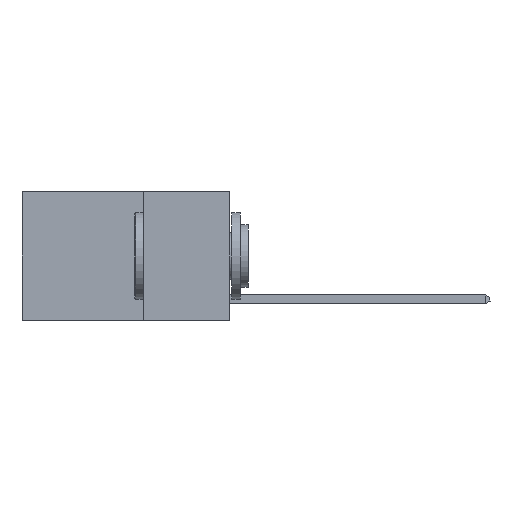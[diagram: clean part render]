
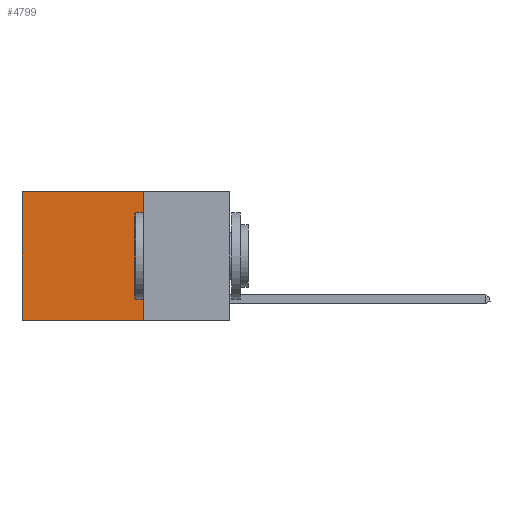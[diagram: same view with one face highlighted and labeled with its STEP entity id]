
A CAD part, left-side view. The second image highlights one B-rep face of the part: STEP entity #4799.
In plain terms, the highlighted planar face has unit normal (-1, 0, 0).
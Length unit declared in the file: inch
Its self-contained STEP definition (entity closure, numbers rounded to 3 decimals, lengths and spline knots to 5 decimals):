
#296 = VECTOR ( 'NONE', #12568, 39.37008 ) ;
#730 = CARTESIAN_POINT ( 'NONE',  ( 0.2625, 0.6, -0.37 ) ) ;
#2338 = AXIS2_PLACEMENT_3D ( 'NONE', #14962, #16241, #8760 ) ;
#2897 = ORIENTED_EDGE ( 'NONE', *, *, #5451, .F. ) ;
#3320 = EDGE_CURVE ( 'NONE', #3560, #9459, #6565, .T. ) ;
#3560 = VERTEX_POINT ( 'NONE', #15603 ) ;
#4278 = LINE ( 'NONE', #8860, #296 ) ;
#4799 = ADVANCED_FACE ( 'NONE', ( #6211 ), #6296, .F. ) ;
#4835 = DIRECTION ( 'NONE',  ( 0., 0., -1. ) ) ;
#5451 = EDGE_CURVE ( 'NONE', #9459, #14580, #12503, .T. ) ;
#5551 = VECTOR ( 'NONE', #8043, 39.37008 ) ;
#5583 = CARTESIAN_POINT ( 'NONE',  ( 0.2625, 0.25, -0.37 ) ) ;
#6211 = FACE_OUTER_BOUND ( 'NONE', #11367, .T. ) ;
#6296 = PLANE ( 'NONE',  #2338 ) ;
#6335 = CARTESIAN_POINT ( 'NONE',  ( 0.2625, 0.25, -0.37 ) ) ;
#6449 = ORIENTED_EDGE ( 'NONE', *, *, #3320, .F. ) ;
#6565 = LINE ( 'NONE', #7354, #16114 ) ;
#7103 = LINE ( 'NONE', #9688, #9957 ) ;
#7354 = CARTESIAN_POINT ( 'NONE',  ( 0.2625, 0.25, 0. ) ) ;
#8043 = DIRECTION ( 'NONE',  ( 0., 1., 0. ) ) ;
#8760 = DIRECTION ( 'NONE',  ( 0., 0., -1. ) ) ;
#8860 = CARTESIAN_POINT ( 'NONE',  ( 0.2625, 0.25, 0. ) ) ;
#9337 = ORIENTED_EDGE ( 'NONE', *, *, #15679, .T. ) ;
#9459 = VERTEX_POINT ( 'NONE', #6335 ) ;
#9688 = CARTESIAN_POINT ( 'NONE',  ( 0.2625, 0.6, 0. ) ) ;
#9957 = VECTOR ( 'NONE', #10291, 39.37008 ) ;
#10291 = DIRECTION ( 'NONE',  ( 0., 0., -1. ) ) ;
#11367 = EDGE_LOOP ( 'NONE', ( #9337, #2897, #6449, #12998 ) ) ;
#12503 = LINE ( 'NONE', #5583, #5551 ) ;
#12568 = DIRECTION ( 'NONE',  ( 0., 1., 0. ) ) ;
#12605 = VERTEX_POINT ( 'NONE', #14824 ) ;
#12998 = ORIENTED_EDGE ( 'NONE', *, *, #14812, .T. ) ;
#14580 = VERTEX_POINT ( 'NONE', #730 ) ;
#14812 = EDGE_CURVE ( 'NONE', #3560, #12605, #4278, .T. ) ;
#14824 = CARTESIAN_POINT ( 'NONE',  ( 0.2625, 0.6, 0. ) ) ;
#14962 = CARTESIAN_POINT ( 'NONE',  ( 0.2625, 0.25, 0. ) ) ;
#15603 = CARTESIAN_POINT ( 'NONE',  ( 0.2625, 0.25, 0. ) ) ;
#15679 = EDGE_CURVE ( 'NONE', #12605, #14580, #7103, .T. ) ;
#16114 = VECTOR ( 'NONE', #4835, 39.37008 ) ;
#16241 = DIRECTION ( 'NONE',  ( 1., 0., 0. ) ) ;
